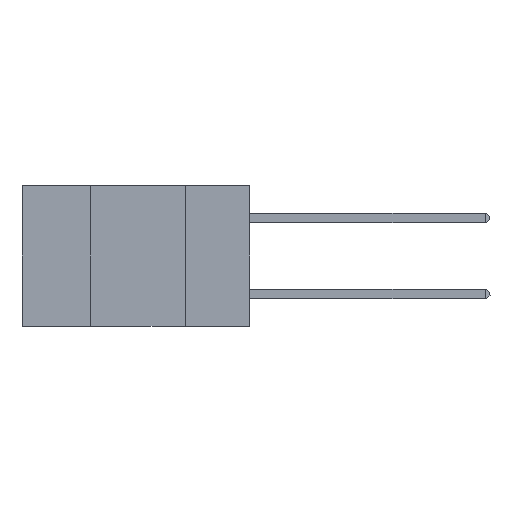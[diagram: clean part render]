
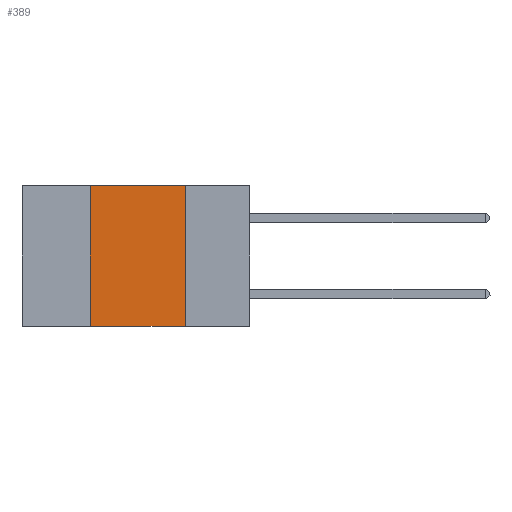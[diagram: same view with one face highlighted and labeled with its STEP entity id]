
A CAD part, left-side view. The second image highlights one B-rep face of the part: STEP entity #389.
In plain terms, the highlighted planar face has unit normal (-1, 0, 0).
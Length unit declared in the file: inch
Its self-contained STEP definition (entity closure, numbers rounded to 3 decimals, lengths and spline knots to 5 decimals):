
#96 = CARTESIAN_POINT ( 'NONE',  ( 0., 0.42, -0.37 ) ) ;
#249 = CARTESIAN_POINT ( 'NONE',  ( 0., 0.17, 0. ) ) ;
#389 = ADVANCED_FACE ( 'NONE', ( #1462 ), #429, .F. ) ;
#392 = LINE ( 'NONE', #2588, #6528 ) ;
#429 = PLANE ( 'NONE',  #702 ) ;
#641 = VECTOR ( 'NONE', #1795, 39.37008 ) ;
#702 = AXIS2_PLACEMENT_3D ( 'NONE', #1827, #8206, #8746 ) ;
#1062 = CARTESIAN_POINT ( 'NONE',  ( 0., 0.17, -0.37 ) ) ;
#1153 = LINE ( 'NONE', #6811, #1346 ) ;
#1331 = VERTEX_POINT ( 'NONE', #96 ) ;
#1346 = VECTOR ( 'NONE', #4063, 39.37008 ) ;
#1430 = ORIENTED_EDGE ( 'NONE', *, *, #4209, .T. ) ;
#1462 = FACE_OUTER_BOUND ( 'NONE', #4810, .T. ) ;
#1628 = CARTESIAN_POINT ( 'NONE',  ( 0., 0.6, -0.37 ) ) ;
#1795 = DIRECTION ( 'NONE',  ( 0., -1., 0. ) ) ;
#1827 = CARTESIAN_POINT ( 'NONE',  ( 0., 0.6, 0. ) ) ;
#2588 = CARTESIAN_POINT ( 'NONE',  ( 0., 0.17, 0. ) ) ;
#2814 = EDGE_CURVE ( 'NONE', #1331, #7438, #1153, .T. ) ;
#3037 = ORIENTED_EDGE ( 'NONE', *, *, #2814, .F. ) ;
#3040 = EDGE_CURVE ( 'NONE', #7438, #8160, #5084, .T. ) ;
#4063 = DIRECTION ( 'NONE',  ( 0., 0., 1. ) ) ;
#4209 = EDGE_CURVE ( 'NONE', #1331, #4484, #8015, .T. ) ;
#4240 = VECTOR ( 'NONE', #5302, 39.37008 ) ;
#4484 = VERTEX_POINT ( 'NONE', #1062 ) ;
#4810 = EDGE_LOOP ( 'NONE', ( #6603, #4873, #3037, #1430 ) ) ;
#4873 = ORIENTED_EDGE ( 'NONE', *, *, #3040, .F. ) ;
#5084 = LINE ( 'NONE', #8462, #641 ) ;
#5302 = DIRECTION ( 'NONE',  ( 0., -1., 0. ) ) ;
#5404 = DIRECTION ( 'NONE',  ( 0., 0., -1. ) ) ;
#6528 = VECTOR ( 'NONE', #5404, 39.37008 ) ;
#6603 = ORIENTED_EDGE ( 'NONE', *, *, #8460, .F. ) ;
#6811 = CARTESIAN_POINT ( 'NONE',  ( 0., 0.42, 0. ) ) ;
#7438 = VERTEX_POINT ( 'NONE', #8849 ) ;
#8015 = LINE ( 'NONE', #1628, #4240 ) ;
#8160 = VERTEX_POINT ( 'NONE', #249 ) ;
#8206 = DIRECTION ( 'NONE',  ( 1., 0., 0. ) ) ;
#8460 = EDGE_CURVE ( 'NONE', #8160, #4484, #392, .T. ) ;
#8462 = CARTESIAN_POINT ( 'NONE',  ( 0., 0.6, 0. ) ) ;
#8746 = DIRECTION ( 'NONE',  ( 0., 0., -1. ) ) ;
#8849 = CARTESIAN_POINT ( 'NONE',  ( 0., 0.42, 0. ) ) ;
